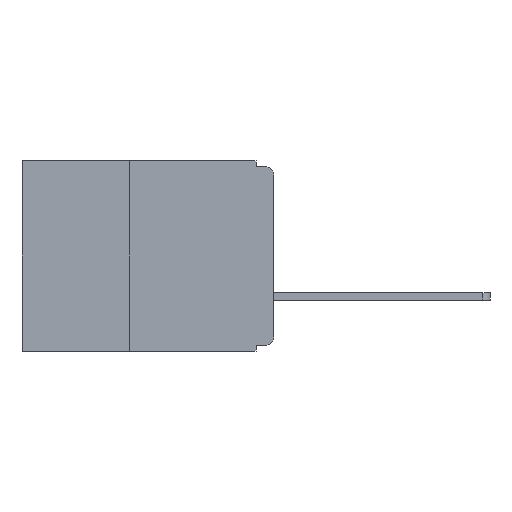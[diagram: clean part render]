
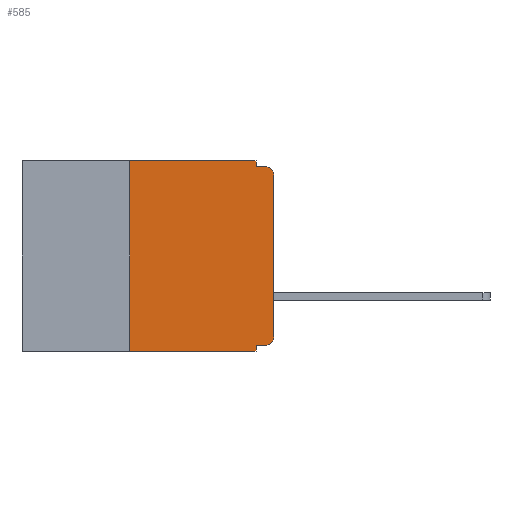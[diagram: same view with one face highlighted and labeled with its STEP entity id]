
A CAD part, left-side view. The second image highlights one B-rep face of the part: STEP entity #585.
In plain terms, the highlighted planar face has unit normal (-1, 0, 0).
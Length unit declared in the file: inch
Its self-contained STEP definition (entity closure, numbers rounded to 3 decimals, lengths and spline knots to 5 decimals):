
#325 = DIRECTION ( 'NONE',  ( -1., 0., 0. ) ) ;
#571 = ORIENTED_EDGE ( 'NONE', *, *, #5254, .F. ) ;
#585 = ADVANCED_FACE ( 'NONE', ( #881 ), #7575, .F. ) ;
#748 = LINE ( 'NONE', #15935, #13481 ) ;
#881 = FACE_OUTER_BOUND ( 'NONE', #6566, .T. ) ;
#1083 = VERTEX_POINT ( 'NONE', #11365 ) ;
#1630 = ORIENTED_EDGE ( 'NONE', *, *, #17907, .F. ) ;
#1860 = DIRECTION ( 'NONE',  ( 0., -1., 0. ) ) ;
#2051 = DIRECTION ( 'NONE',  ( 0., 0., 1. ) ) ;
#2407 = VERTEX_POINT ( 'NONE', #3754 ) ;
#2468 = EDGE_CURVE ( 'NONE', #5110, #13727, #15578, .T. ) ;
#2529 = CARTESIAN_POINT ( 'NONE',  ( 0., 0.437, -0.33 ) ) ;
#2714 = ORIENTED_EDGE ( 'NONE', *, *, #11790, .T. ) ;
#3120 = LINE ( 'NONE', #5753, #19987 ) ;
#3499 = ORIENTED_EDGE ( 'NONE', *, *, #21094, .T. ) ;
#3586 = DIRECTION ( 'NONE',  ( -1., 0., 0. ) ) ;
#3618 = EDGE_CURVE ( 'NONE', #2407, #15938, #19679, .T. ) ;
#3754 = CARTESIAN_POINT ( 'NONE',  ( 0., 0.015, -0.32 ) ) ;
#4124 = VECTOR ( 'NONE', #2051, 39.37008 ) ;
#4374 = VERTEX_POINT ( 'NONE', #19757 ) ;
#4401 = VERTEX_POINT ( 'NONE', #17370 ) ;
#4760 = CIRCLE ( 'NONE', #5100, 0.015 ) ;
#4926 = DIRECTION ( 'NONE',  ( 0., -1., 0. ) ) ;
#5100 = AXIS2_PLACEMENT_3D ( 'NONE', #13468, #3586, #15086 ) ;
#5110 = VERTEX_POINT ( 'NONE', #18629 ) ;
#5163 = LINE ( 'NONE', #13642, #4124 ) ;
#5254 = EDGE_CURVE ( 'NONE', #17332, #1083, #6094, .T. ) ;
#5589 = VECTOR ( 'NONE', #17340, 39.37008 ) ;
#5595 = ORIENTED_EDGE ( 'NONE', *, *, #16679, .F. ) ;
#5753 = CARTESIAN_POINT ( 'NONE',  ( 0., 0.031, 0. ) ) ;
#5996 = CARTESIAN_POINT ( 'NONE',  ( 0., 0., -0.025 ) ) ;
#6094 = LINE ( 'NONE', #16901, #5589 ) ;
#6566 = EDGE_LOOP ( 'NONE', ( #20337, #3499, #571, #5595, #9986, #1630, #14843, #19111, #15332, #2714 ) ) ;
#7031 = DIRECTION ( 'NONE',  ( 0., 0., -1. ) ) ;
#7059 = DIRECTION ( 'NONE',  ( 1., 0., 0. ) ) ;
#7550 = CARTESIAN_POINT ( 'NONE',  ( 0., 0.437, 0. ) ) ;
#7575 = PLANE ( 'NONE',  #19526 ) ;
#7726 = CARTESIAN_POINT ( 'NONE',  ( 0., 0.031, -0.01 ) ) ;
#9577 = VERTEX_POINT ( 'NONE', #5996 ) ;
#9986 = ORIENTED_EDGE ( 'NONE', *, *, #20043, .F. ) ;
#10334 = CARTESIAN_POINT ( 'NONE',  ( 0., 0.015, -0.025 ) ) ;
#10736 = DIRECTION ( 'NONE',  ( 0., 0., -1. ) ) ;
#10771 = CARTESIAN_POINT ( 'NONE',  ( 0., 0., 0. ) ) ;
#11254 = VECTOR ( 'NONE', #1860, 39.37008 ) ;
#11350 = EDGE_CURVE ( 'NONE', #4374, #9577, #13533, .T. ) ;
#11365 = CARTESIAN_POINT ( 'NONE',  ( 0., 0.015, -0.01 ) ) ;
#11790 = EDGE_CURVE ( 'NONE', #2407, #4374, #4760, .T. ) ;
#11965 = DIRECTION ( 'NONE',  ( 0., 0., -1. ) ) ;
#12384 = VERTEX_POINT ( 'NONE', #17897 ) ;
#12412 = AXIS2_PLACEMENT_3D ( 'NONE', #10334, #325, #11965 ) ;
#13468 = CARTESIAN_POINT ( 'NONE',  ( 0., 0.015, -0.305 ) ) ;
#13481 = VECTOR ( 'NONE', #17556, 39.37008 ) ;
#13533 = LINE ( 'NONE', #10771, #18330 ) ;
#13642 = CARTESIAN_POINT ( 'NONE',  ( 0., 0.25, -0.33 ) ) ;
#13727 = VERTEX_POINT ( 'NONE', #19661 ) ;
#14843 = ORIENTED_EDGE ( 'NONE', *, *, #2468, .T. ) ;
#15086 = DIRECTION ( 'NONE',  ( 0., 0., -1. ) ) ;
#15332 = ORIENTED_EDGE ( 'NONE', *, *, #3618, .F. ) ;
#15411 = VECTOR ( 'NONE', #18729, 39.37008 ) ;
#15566 = VECTOR ( 'NONE', #4926, 39.37008 ) ;
#15578 = LINE ( 'NONE', #2529, #11254 ) ;
#15935 = CARTESIAN_POINT ( 'NONE',  ( 0., 0.031, -0.33 ) ) ;
#15938 = VERTEX_POINT ( 'NONE', #17062 ) ;
#16067 = LINE ( 'NONE', #21126, #15566 ) ;
#16114 = EDGE_CURVE ( 'NONE', #15938, #13727, #748, .T. ) ;
#16679 = EDGE_CURVE ( 'NONE', #12384, #17332, #3120, .T. ) ;
#16901 = CARTESIAN_POINT ( 'NONE',  ( 0., 0., -0.01 ) ) ;
#17062 = CARTESIAN_POINT ( 'NONE',  ( 0., 0.031, -0.32 ) ) ;
#17332 = VERTEX_POINT ( 'NONE', #7726 ) ;
#17340 = DIRECTION ( 'NONE',  ( 0., -1., 0. ) ) ;
#17370 = CARTESIAN_POINT ( 'NONE',  ( 0., 0.25, 0. ) ) ;
#17556 = DIRECTION ( 'NONE',  ( 0., 0., -1. ) ) ;
#17897 = CARTESIAN_POINT ( 'NONE',  ( 0., 0.031, 0. ) ) ;
#17907 = EDGE_CURVE ( 'NONE', #5110, #4401, #5163, .T. ) ;
#18330 = VECTOR ( 'NONE', #20424, 39.37008 ) ;
#18629 = CARTESIAN_POINT ( 'NONE',  ( 0., 0.25, -0.33 ) ) ;
#18633 = CARTESIAN_POINT ( 'NONE',  ( 0., 0., -0.32 ) ) ;
#18663 = CIRCLE ( 'NONE', #12412, 0.015 ) ;
#18729 = DIRECTION ( 'NONE',  ( 0., 1., 0. ) ) ;
#19111 = ORIENTED_EDGE ( 'NONE', *, *, #16114, .F. ) ;
#19526 = AXIS2_PLACEMENT_3D ( 'NONE', #7550, #7059, #7031 ) ;
#19661 = CARTESIAN_POINT ( 'NONE',  ( 0., 0.031, -0.33 ) ) ;
#19679 = LINE ( 'NONE', #18633, #15411 ) ;
#19757 = CARTESIAN_POINT ( 'NONE',  ( 0., 0., -0.305 ) ) ;
#19987 = VECTOR ( 'NONE', #10736, 39.37008 ) ;
#20043 = EDGE_CURVE ( 'NONE', #4401, #12384, #16067, .T. ) ;
#20337 = ORIENTED_EDGE ( 'NONE', *, *, #11350, .T. ) ;
#20424 = DIRECTION ( 'NONE',  ( 0., 0., 1. ) ) ;
#21094 = EDGE_CURVE ( 'NONE', #9577, #1083, #18663, .T. ) ;
#21126 = CARTESIAN_POINT ( 'NONE',  ( 0., 0.437, 0. ) ) ;
